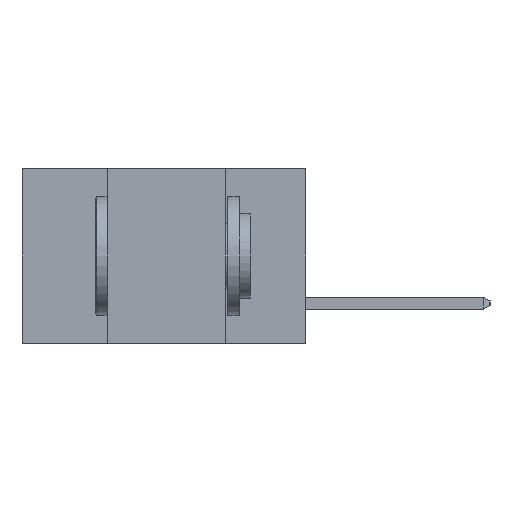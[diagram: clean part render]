
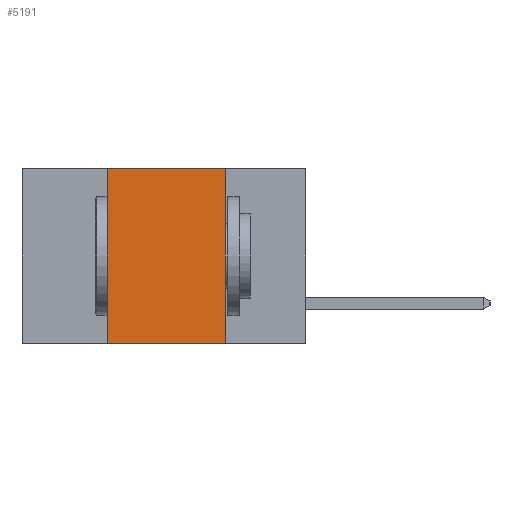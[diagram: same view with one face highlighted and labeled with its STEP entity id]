
A CAD part, left-side view. The second image highlights one B-rep face of the part: STEP entity #5191.
In plain terms, the highlighted planar face has unit normal (-1, 0, 0).
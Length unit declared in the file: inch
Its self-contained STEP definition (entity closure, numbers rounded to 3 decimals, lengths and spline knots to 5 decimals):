
#112 = VERTEX_POINT ( 'NONE', #16396 ) ;
#366 = VECTOR ( 'NONE', #10520, 39.37008 ) ;
#598 = CARTESIAN_POINT ( 'NONE',  ( 0., 0.42, 0. ) ) ;
#850 = VERTEX_POINT ( 'NONE', #6987 ) ;
#1709 = VECTOR ( 'NONE', #2011, 39.37008 ) ;
#1940 = ORIENTED_EDGE ( 'NONE', *, *, #16217, .F. ) ;
#2011 = DIRECTION ( 'NONE',  ( 0., 0., 1. ) ) ;
#2555 = EDGE_LOOP ( 'NONE', ( #4440, #1940, #9992, #9052 ) ) ;
#3955 = CARTESIAN_POINT ( 'NONE',  ( 0., 0.6, 0. ) ) ;
#4440 = ORIENTED_EDGE ( 'NONE', *, *, #5909, .F. ) ;
#4467 = LINE ( 'NONE', #5253, #366 ) ;
#4913 = LINE ( 'NONE', #598, #1709 ) ;
#5191 = ADVANCED_FACE ( 'NONE', ( #14508 ), #10523, .F. ) ;
#5253 = CARTESIAN_POINT ( 'NONE',  ( 0., 0.6, -0.37 ) ) ;
#5791 = VECTOR ( 'NONE', #10561, 39.37008 ) ;
#5909 = EDGE_CURVE ( 'NONE', #850, #112, #9129, .T. ) ;
#5925 = VERTEX_POINT ( 'NONE', #8327 ) ;
#6987 = CARTESIAN_POINT ( 'NONE',  ( 0., 0.17, 0. ) ) ;
#7694 = EDGE_CURVE ( 'NONE', #7711, #5925, #4913, .T. ) ;
#7711 = VERTEX_POINT ( 'NONE', #12690 ) ;
#8327 = CARTESIAN_POINT ( 'NONE',  ( 0., 0.42, 0. ) ) ;
#8592 = EDGE_CURVE ( 'NONE', #7711, #112, #4467, .T. ) ;
#9052 = ORIENTED_EDGE ( 'NONE', *, *, #8592, .T. ) ;
#9129 = LINE ( 'NONE', #10250, #12630 ) ;
#9992 = ORIENTED_EDGE ( 'NONE', *, *, #7694, .F. ) ;
#10250 = CARTESIAN_POINT ( 'NONE',  ( 0., 0.17, 0. ) ) ;
#10290 = DIRECTION ( 'NONE',  ( 0., 0., -1. ) ) ;
#10311 = AXIS2_PLACEMENT_3D ( 'NONE', #10539, #12326, #12304 ) ;
#10520 = DIRECTION ( 'NONE',  ( 0., -1., 0. ) ) ;
#10523 = PLANE ( 'NONE',  #10311 ) ;
#10539 = CARTESIAN_POINT ( 'NONE',  ( 0., 0.6, 0. ) ) ;
#10561 = DIRECTION ( 'NONE',  ( 0., -1., 0. ) ) ;
#12304 = DIRECTION ( 'NONE',  ( 0., 0., -1. ) ) ;
#12326 = DIRECTION ( 'NONE',  ( 1., 0., 0. ) ) ;
#12630 = VECTOR ( 'NONE', #10290, 39.37008 ) ;
#12690 = CARTESIAN_POINT ( 'NONE',  ( 0., 0.42, -0.37 ) ) ;
#12840 = LINE ( 'NONE', #3955, #5791 ) ;
#14508 = FACE_OUTER_BOUND ( 'NONE', #2555, .T. ) ;
#16217 = EDGE_CURVE ( 'NONE', #5925, #850, #12840, .T. ) ;
#16396 = CARTESIAN_POINT ( 'NONE',  ( 0., 0.17, -0.37 ) ) ;
